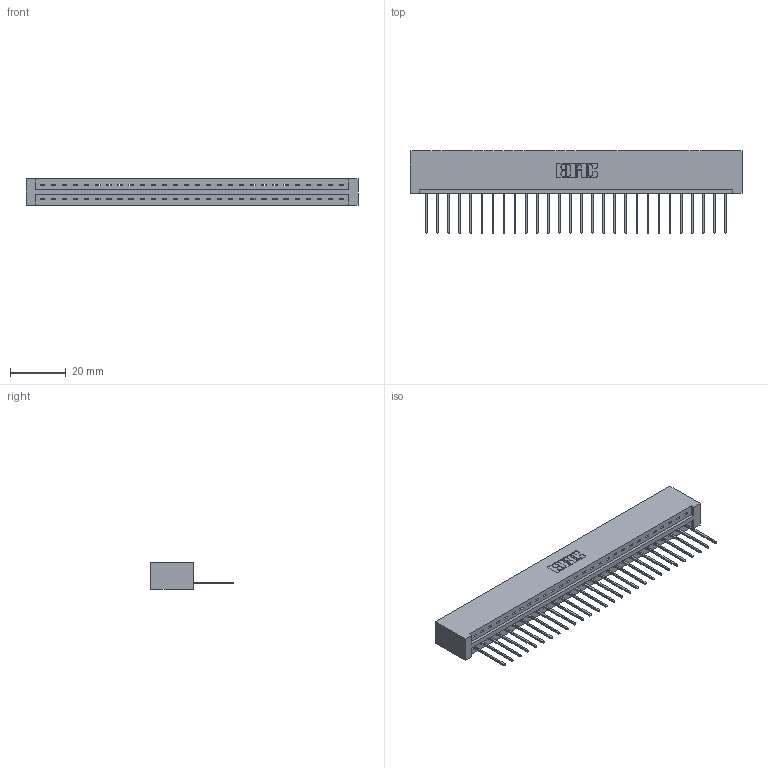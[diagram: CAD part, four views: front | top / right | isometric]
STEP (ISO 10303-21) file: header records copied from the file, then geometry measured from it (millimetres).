
FILE_DESCRIPTION (( 'STEP AP203' ), '1' );
FILE_NAME ('337-028-540-101.STEP', '2018-08-06T10:17:40', ( '' ), ( '' ), 'SwSTEP 2.0', 'SolidWorks 2016', '' );
FILE_SCHEMA (( 'CONFIG_CONTROL_DESIGN' ));
Length unit declared in the file: inch
Products named in the file (3): 337 Part_No Mounting Lugs; 345-292-001_345-293-140; 337-028-540-101
Assembly tree (29 placements, depth 2):
  337-028-540-101
    337 Part_No Mounting Lugs
    345-292-001_345-293-140  x28
Bounding box: 118.82 x 29.47 x 9.4 mm (x, y, z)
Volume: 12950.9 mm3; surface area: 13568 mm2
Topology: 29 solids, 29 shells, 1842 faces, 5551 edges, 3662 vertices
Faces by surface type: plane 1354, cylinder 488
Entity records: 22365 total; most frequent: CARTESIAN_POINT 3902, ORIENTED_EDGE 3866, DIRECTION 3305, EDGE_CURVE 1933, VECTOR 1813, LINE 1813, VERTEX_POINT 1286, AXIS2_PLACEMENT_3D 746
